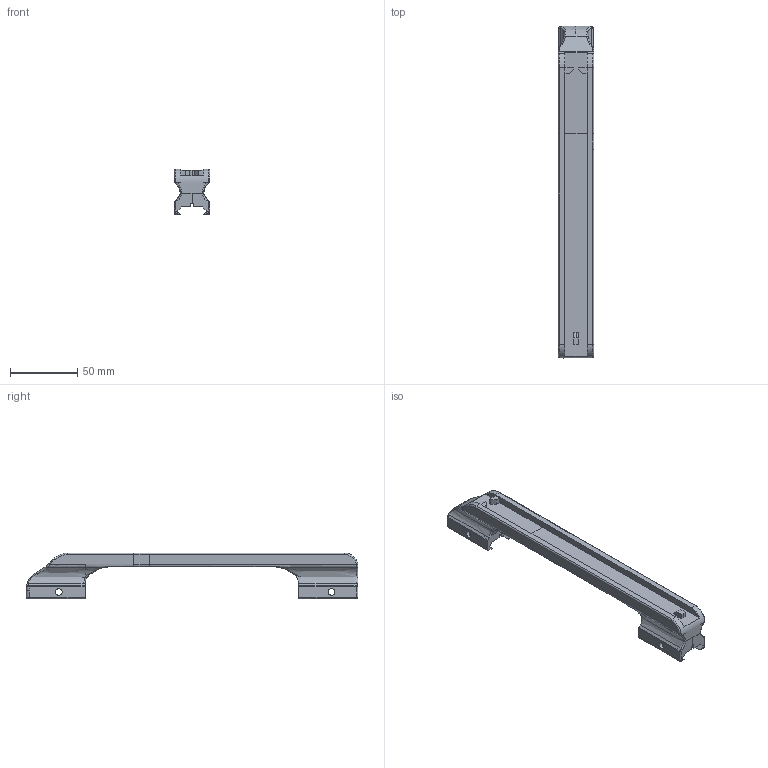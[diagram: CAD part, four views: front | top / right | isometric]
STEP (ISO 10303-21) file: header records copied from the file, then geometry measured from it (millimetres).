
FILE_DESCRIPTION(/* description */ (''),/* implementation_level */ '2;1');
FILE_NAME(/* name */ 'SG22 Carry Handle No Optic Release.step',/* time_stamp */ '2021-03-18T09:36:23-06:00',/* author */ (''),/* organization */ (''),/* preprocessor_version */ 'ST-DEVELOPER v18.1',/* originating_system */ 'Autodesk Translation Framework v9.10.0.1330',/* authorisation */ '');
FILE_SCHEMA (('AUTOMOTIVE_DESIGN { 1 0 10303 214 3 1 1 }'));
Length unit declared in the file: inch
Products named in the file (1): Space Gun Beta Ready
Bounding box: 26.42 x 246.43 x 34.01 mm (x, y, z)
Volume: 79855.3 mm3; surface area: 27435.7 mm2
Topology: 1 solids, 1 shells, 344 faces, 960 edges, 613 vertices
Faces by surface type: plane 204, bspline 78, cylinder 50, torus 6, sphere 6
Full cylindrical faces by diameter (mm): 5 x4
Entity records: 13023 total; most frequent: CARTESIAN_POINT 4604, ORIENTED_EDGE 1916, DIRECTION 1494, EDGE_CURVE 958, VERTEX_POINT 613, LINE 580, VECTOR 580, AXIS2_PLACEMENT_3D 457
